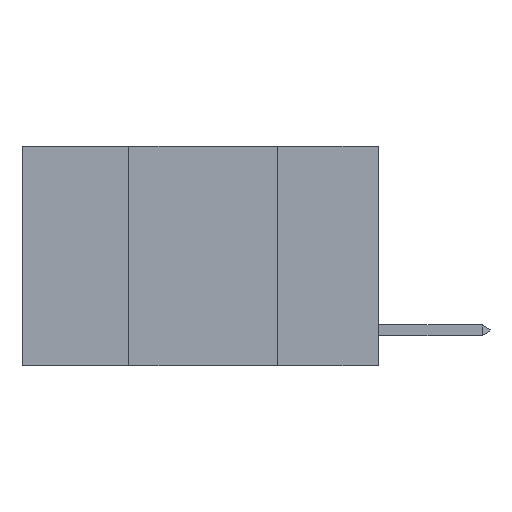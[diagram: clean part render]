
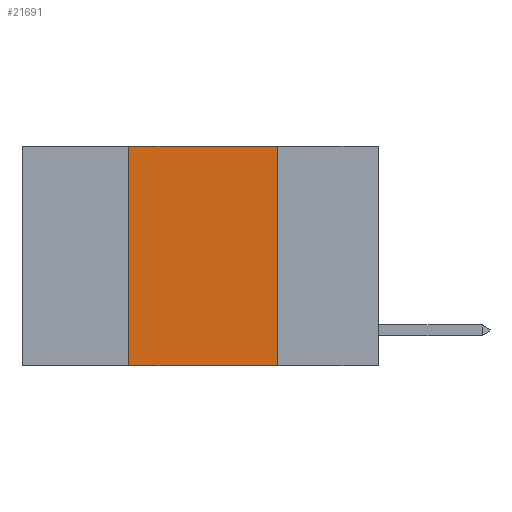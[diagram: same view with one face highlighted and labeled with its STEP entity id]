
A CAD part, left-side view. The second image highlights one B-rep face of the part: STEP entity #21691.
In plain terms, the highlighted planar face has unit normal (-1, 0, 0).
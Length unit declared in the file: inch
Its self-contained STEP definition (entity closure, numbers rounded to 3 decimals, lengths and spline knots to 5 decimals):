
#370 = DIRECTION ( 'NONE',  ( 0., 0., -1. ) ) ;
#876 = DIRECTION ( 'NONE',  ( 0., -1., 0. ) ) ;
#1621 = VERTEX_POINT ( 'NONE', #18677 ) ;
#3500 = LINE ( 'NONE', #12938, #13437 ) ;
#3564 = VECTOR ( 'NONE', #876, 39.37008 ) ;
#4070 = CARTESIAN_POINT ( 'NONE',  ( 0., 0.17, -0.37 ) ) ;
#5079 = VERTEX_POINT ( 'NONE', #4070 ) ;
#5112 = LINE ( 'NONE', #22933, #14429 ) ;
#7168 = AXIS2_PLACEMENT_3D ( 'NONE', #10261, #12243, #370 ) ;
#8537 = ORIENTED_EDGE ( 'NONE', *, *, #9979, .F. ) ;
#9526 = LINE ( 'NONE', #14709, #3564 ) ;
#9633 = CARTESIAN_POINT ( 'NONE',  ( 0., 0.17, 0. ) ) ;
#9763 = ORIENTED_EDGE ( 'NONE', *, *, #23730, .T. ) ;
#9979 = EDGE_CURVE ( 'NONE', #22945, #20839, #5112, .T. ) ;
#10261 = CARTESIAN_POINT ( 'NONE',  ( 0., 0.6, 0. ) ) ;
#10348 = EDGE_CURVE ( 'NONE', #20839, #5079, #12885, .T. ) ;
#11157 = EDGE_CURVE ( 'NONE', #1621, #22945, #3500, .T. ) ;
#12243 = DIRECTION ( 'NONE',  ( 1., 0., 0. ) ) ;
#12885 = LINE ( 'NONE', #22083, #16880 ) ;
#12938 = CARTESIAN_POINT ( 'NONE',  ( 0., 0.42, 0. ) ) ;
#13133 = ORIENTED_EDGE ( 'NONE', *, *, #10348, .F. ) ;
#13241 = DIRECTION ( 'NONE',  ( 0., -1., 0. ) ) ;
#13437 = VECTOR ( 'NONE', #14917, 39.37008 ) ;
#14429 = VECTOR ( 'NONE', #13241, 39.37008 ) ;
#14709 = CARTESIAN_POINT ( 'NONE',  ( 0., 0.6, -0.37 ) ) ;
#14917 = DIRECTION ( 'NONE',  ( 0., 0., 1. ) ) ;
#16310 = EDGE_LOOP ( 'NONE', ( #13133, #8537, #24641, #9763 ) ) ;
#16880 = VECTOR ( 'NONE', #18301, 39.37008 ) ;
#18301 = DIRECTION ( 'NONE',  ( 0., 0., -1. ) ) ;
#18677 = CARTESIAN_POINT ( 'NONE',  ( 0., 0.42, -0.37 ) ) ;
#20036 = CARTESIAN_POINT ( 'NONE',  ( 0., 0.42, 0. ) ) ;
#20839 = VERTEX_POINT ( 'NONE', #9633 ) ;
#21691 = ADVANCED_FACE ( 'NONE', ( #22751 ), #21955, .F. ) ;
#21955 = PLANE ( 'NONE',  #7168 ) ;
#22083 = CARTESIAN_POINT ( 'NONE',  ( 0., 0.17, 0. ) ) ;
#22751 = FACE_OUTER_BOUND ( 'NONE', #16310, .T. ) ;
#22933 = CARTESIAN_POINT ( 'NONE',  ( 0., 0.6, 0. ) ) ;
#22945 = VERTEX_POINT ( 'NONE', #20036 ) ;
#23730 = EDGE_CURVE ( 'NONE', #1621, #5079, #9526, .T. ) ;
#24641 = ORIENTED_EDGE ( 'NONE', *, *, #11157, .F. ) ;
